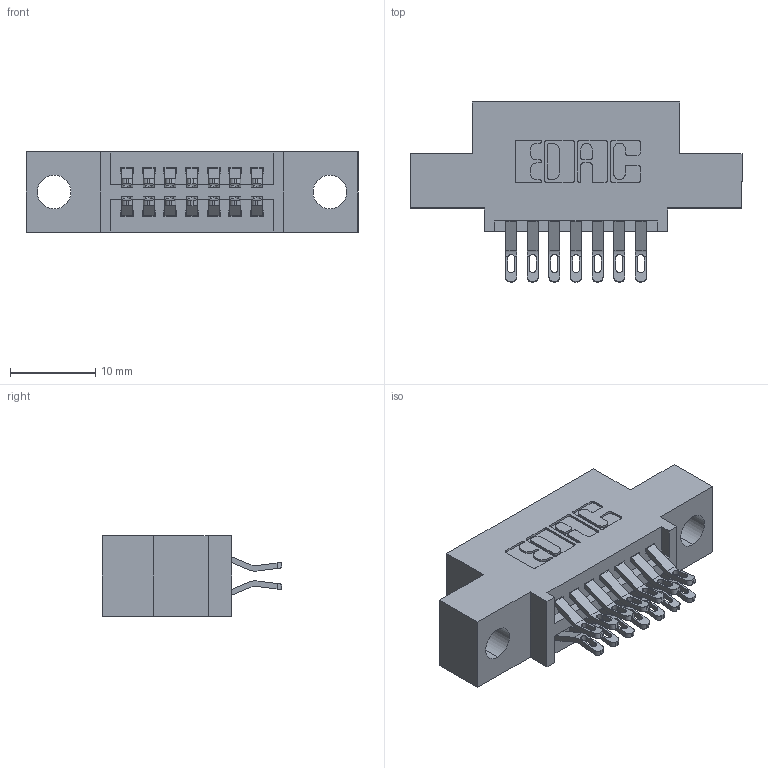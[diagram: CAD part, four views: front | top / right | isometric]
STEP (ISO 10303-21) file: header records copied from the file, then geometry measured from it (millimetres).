
FILE_DESCRIPTION (( 'STEP AP203' ), '1' );
FILE_NAME ('345-014-555-504.STEP', '2021-05-19T16:05:56', ( '' ), ( '' ), 'SwSTEP 2.0', 'SolidWorks 2020', '' );
FILE_SCHEMA (( 'CONFIG_CONTROL_DESIGN' ));
Length unit declared in the file: inch
Products named in the file (3): 345-014-555-504; 345 Part_0.110 Offset - 0.156 Dia-TI; 345-292-001_555 Tail
Assembly tree (15 placements, depth 2):
  345-014-555-504
    345 Part_0.110 Offset - 0.156 Dia-TI
    345-292-001_555 Tail  x14
Bounding box: 38.99 x 21.13 x 9.4 mm (x, y, z)
Volume: 3323.8 mm3; surface area: 4321 mm2
Topology: 15 solids, 15 shells, 928 faces, 2867 edges, 1910 vertices
Faces by surface type: plane 532, cylinder 396
Entity records: 11081 total; most frequent: CARTESIAN_POINT 1932, ORIENTED_EDGE 1834, DIRECTION 1713, EDGE_CURVE 917, VECTOR 737, LINE 737, VERTEX_POINT 610, AXIS2_PLACEMENT_3D 488
